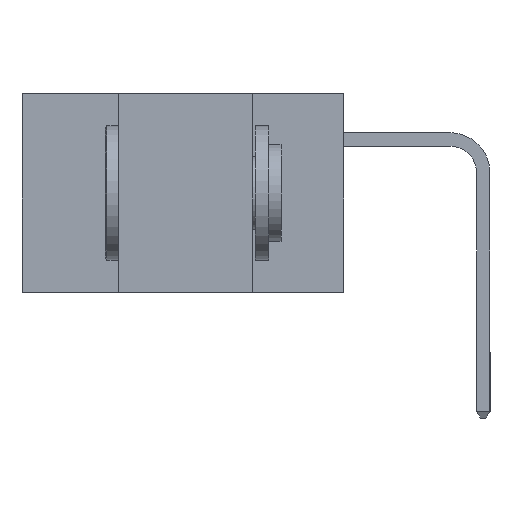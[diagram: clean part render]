
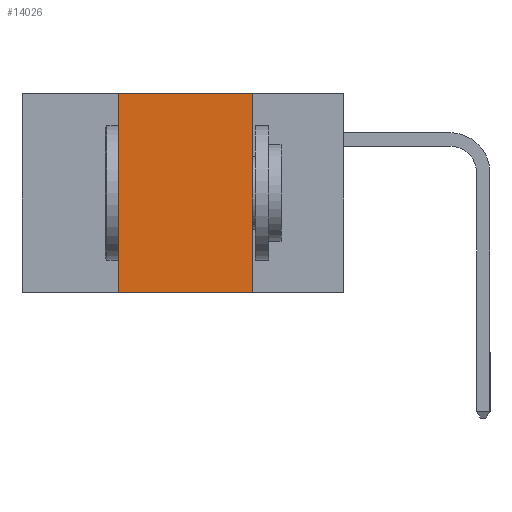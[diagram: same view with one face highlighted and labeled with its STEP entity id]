
A CAD part, left-side view. The second image highlights one B-rep face of the part: STEP entity #14026.
In plain terms, the highlighted planar face has unit normal (-1, 0, 0).
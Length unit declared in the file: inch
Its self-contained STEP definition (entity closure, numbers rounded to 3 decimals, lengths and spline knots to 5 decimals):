
#187 = AXIS2_PLACEMENT_3D ( 'NONE', #767, #3241, #8185 ) ;
#303 = CARTESIAN_POINT ( 'NONE',  ( 0., 0.42, -0.37 ) ) ;
#395 = DIRECTION ( 'NONE',  ( 0., 0., -1. ) ) ;
#767 = CARTESIAN_POINT ( 'NONE',  ( 0., 0.6, 0. ) ) ;
#1425 = LINE ( 'NONE', #7720, #3020 ) ;
#1946 = FACE_OUTER_BOUND ( 'NONE', #4095, .T. ) ;
#2038 = VECTOR ( 'NONE', #10592, 39.37008 ) ;
#2601 = CARTESIAN_POINT ( 'NONE',  ( 0., 0.17, -0.37 ) ) ;
#3020 = VECTOR ( 'NONE', #395, 39.37008 ) ;
#3241 = DIRECTION ( 'NONE',  ( 1., 0., 0. ) ) ;
#3329 = EDGE_CURVE ( 'NONE', #13246, #5525, #1425, .T. ) ;
#3810 = EDGE_CURVE ( 'NONE', #6182, #9673, #8777, .T. ) ;
#4095 = EDGE_LOOP ( 'NONE', ( #4679, #10294, #13342, #11569 ) ) ;
#4679 = ORIENTED_EDGE ( 'NONE', *, *, #3329, .F. ) ;
#5525 = VERTEX_POINT ( 'NONE', #2601 ) ;
#5651 = CARTESIAN_POINT ( 'NONE',  ( 0., 0.6, 0. ) ) ;
#6182 = VERTEX_POINT ( 'NONE', #14278 ) ;
#6713 = CARTESIAN_POINT ( 'NONE',  ( 0., 0.6, -0.37 ) ) ;
#6926 = VECTOR ( 'NONE', #7622, 39.37008 ) ;
#7622 = DIRECTION ( 'NONE',  ( 0., 0., 1. ) ) ;
#7720 = CARTESIAN_POINT ( 'NONE',  ( 0., 0.17, -0.37 ) ) ;
#8185 = DIRECTION ( 'NONE',  ( 0., 0., -1. ) ) ;
#8557 = CARTESIAN_POINT ( 'NONE',  ( 0., 0.17, 0. ) ) ;
#8777 = LINE ( 'NONE', #303, #6926 ) ;
#9673 = VERTEX_POINT ( 'NONE', #13376 ) ;
#10294 = ORIENTED_EDGE ( 'NONE', *, *, #12206, .F. ) ;
#10592 = DIRECTION ( 'NONE',  ( 0., -1., 0. ) ) ;
#11540 = EDGE_CURVE ( 'NONE', #6182, #5525, #12899, .T. ) ;
#11569 = ORIENTED_EDGE ( 'NONE', *, *, #11540, .T. ) ;
#11848 = PLANE ( 'NONE',  #187 ) ;
#12206 = EDGE_CURVE ( 'NONE', #9673, #13246, #12957, .T. ) ;
#12899 = LINE ( 'NONE', #6713, #14673 ) ;
#12957 = LINE ( 'NONE', #5651, #2038 ) ;
#13246 = VERTEX_POINT ( 'NONE', #8557 ) ;
#13342 = ORIENTED_EDGE ( 'NONE', *, *, #3810, .F. ) ;
#13376 = CARTESIAN_POINT ( 'NONE',  ( 0., 0.42, 0. ) ) ;
#14026 = ADVANCED_FACE ( 'NONE', ( #1946 ), #11848, .F. ) ;
#14278 = CARTESIAN_POINT ( 'NONE',  ( 0., 0.42, -0.37 ) ) ;
#14673 = VECTOR ( 'NONE', #15220, 39.37008 ) ;
#15220 = DIRECTION ( 'NONE',  ( 0., -1., 0. ) ) ;
